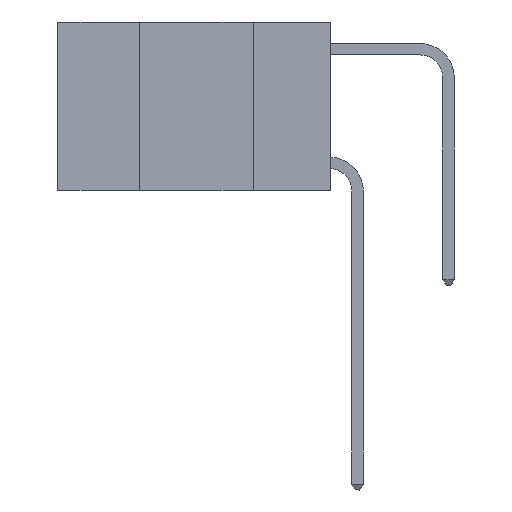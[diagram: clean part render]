
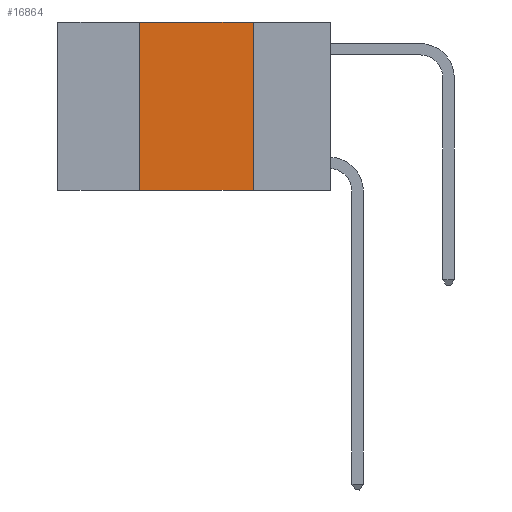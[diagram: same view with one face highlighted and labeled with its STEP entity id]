
A CAD part, left-side view. The second image highlights one B-rep face of the part: STEP entity #16864.
In plain terms, the highlighted planar face has unit normal (-1, 0, 0).
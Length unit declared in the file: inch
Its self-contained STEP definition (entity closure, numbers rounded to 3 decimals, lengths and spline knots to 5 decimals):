
#429 = EDGE_CURVE ( 'NONE', #7758, #24535, #3049, .T. ) ;
#1374 = CARTESIAN_POINT ( 'NONE',  ( 0., 0.17, 0. ) ) ;
#1395 = ORIENTED_EDGE ( 'NONE', *, *, #25759, .F. ) ;
#3049 = LINE ( 'NONE', #7809, #7352 ) ;
#3111 = LINE ( 'NONE', #27087, #18637 ) ;
#3884 = DIRECTION ( 'NONE',  ( 0., 0., -1. ) ) ;
#4425 = ORIENTED_EDGE ( 'NONE', *, *, #429, .F. ) ;
#4641 = VERTEX_POINT ( 'NONE', #1374 ) ;
#4823 = CARTESIAN_POINT ( 'NONE',  ( 0., 0.6, -0.37 ) ) ;
#7049 = DIRECTION ( 'NONE',  ( 0., -1., 0. ) ) ;
#7204 = DIRECTION ( 'NONE',  ( 0., -1., 0. ) ) ;
#7212 = CARTESIAN_POINT ( 'NONE',  ( 0., 0.6, 0. ) ) ;
#7352 = VECTOR ( 'NONE', #27119, 39.37008 ) ;
#7758 = VERTEX_POINT ( 'NONE', #24674 ) ;
#7809 = CARTESIAN_POINT ( 'NONE',  ( 0., 0.42, 0. ) ) ;
#9117 = LINE ( 'NONE', #13546, #25263 ) ;
#10488 = LINE ( 'NONE', #4823, #26605 ) ;
#11412 = DIRECTION ( 'NONE',  ( 1., 0., 0. ) ) ;
#12273 = EDGE_CURVE ( 'NONE', #7758, #15777, #10488, .T. ) ;
#12890 = EDGE_LOOP ( 'NONE', ( #1395, #19298, #4425, #16061 ) ) ;
#13058 = EDGE_CURVE ( 'NONE', #24535, #4641, #9117, .T. ) ;
#13546 = CARTESIAN_POINT ( 'NONE',  ( 0., 0.6, 0. ) ) ;
#14568 = CARTESIAN_POINT ( 'NONE',  ( 0., 0.42, 0. ) ) ;
#15777 = VERTEX_POINT ( 'NONE', #25654 ) ;
#16061 = ORIENTED_EDGE ( 'NONE', *, *, #12273, .T. ) ;
#16864 = ADVANCED_FACE ( 'NONE', ( #19186 ), #24087, .F. ) ;
#18637 = VECTOR ( 'NONE', #3884, 39.37008 ) ;
#19186 = FACE_OUTER_BOUND ( 'NONE', #12890, .T. ) ;
#19298 = ORIENTED_EDGE ( 'NONE', *, *, #13058, .F. ) ;
#20187 = AXIS2_PLACEMENT_3D ( 'NONE', #7212, #11412, #26158 ) ;
#24087 = PLANE ( 'NONE',  #20187 ) ;
#24535 = VERTEX_POINT ( 'NONE', #14568 ) ;
#24674 = CARTESIAN_POINT ( 'NONE',  ( 0., 0.42, -0.37 ) ) ;
#25263 = VECTOR ( 'NONE', #7204, 39.37008 ) ;
#25654 = CARTESIAN_POINT ( 'NONE',  ( 0., 0.17, -0.37 ) ) ;
#25759 = EDGE_CURVE ( 'NONE', #4641, #15777, #3111, .T. ) ;
#26158 = DIRECTION ( 'NONE',  ( 0., 0., -1. ) ) ;
#26605 = VECTOR ( 'NONE', #7049, 39.37008 ) ;
#27087 = CARTESIAN_POINT ( 'NONE',  ( 0., 0.17, 0. ) ) ;
#27119 = DIRECTION ( 'NONE',  ( 0., 0., 1. ) ) ;
